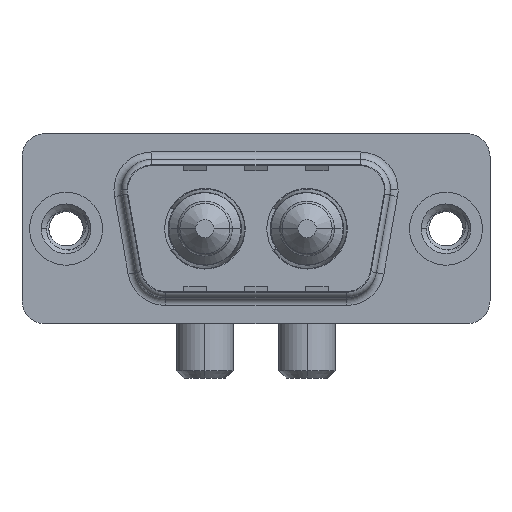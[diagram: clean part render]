
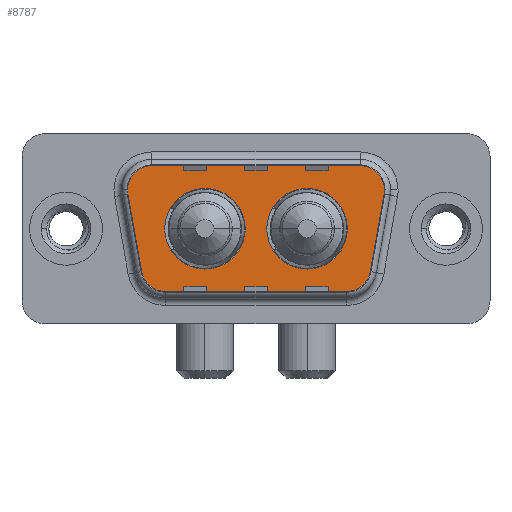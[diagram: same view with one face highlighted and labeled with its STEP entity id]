
A CAD part, top view. The second image highlights one B-rep face of the part: STEP entity #8787.
In plain terms, the highlighted planar face has unit normal (0, 0, 1).
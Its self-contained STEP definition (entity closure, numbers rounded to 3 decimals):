
#84 = CARTESIAN_POINT ( 'NONE',  ( 9.14, 0., 0. ) ) ;
#316 = LINE ( 'NONE', #6560, #7361 ) ;
#376 = CIRCLE ( 'NONE', #4851, 2.65 ) ;
#379 = DIRECTION ( 'NONE',  ( 0., 0., 1. ) ) ;
#532 = VERTEX_POINT ( 'NONE', #5671 ) ;
#815 = VECTOR ( 'NONE', #4176, 1000. ) ;
#820 = EDGE_CURVE ( 'NONE', #9684, #3343, #3651, .T. ) ;
#829 = EDGE_LOOP ( 'NONE', ( #10375, #3904, #11262, #5884, #11087, #3032, #9886, #11338, #3452 ) ) ;
#859 = DIRECTION ( 'NONE',  ( -1., 0., 0. ) ) ;
#915 = DIRECTION ( 'NONE',  ( 0., 0., 1. ) ) ;
#1034 = DIRECTION ( 'NONE',  ( 1., 0., 0. ) ) ;
#1186 = CARTESIAN_POINT ( 'NONE',  ( 5.436, 4.9, 0. ) ) ;
#1295 = EDGE_CURVE ( 'NONE', #2386, #5012, #4028, .T. ) ;
#1323 = CIRCLE ( 'NONE', #1509, 2.65 ) ;
#1374 = CARTESIAN_POINT ( 'NONE',  ( 3.466, 2.553, 0. ) ) ;
#1493 = ORIENTED_EDGE ( 'NONE', *, *, #3685, .F. ) ;
#1509 = AXIS2_PLACEMENT_3D ( 'NONE', #84, #6387, #7388 ) ;
#1539 = AXIS2_PLACEMENT_3D ( 'NONE', #5334, #1946, #9095 ) ;
#1560 = VECTOR ( 'NONE', #4746, 1000. ) ;
#1610 = DIRECTION ( 'NONE',  ( 0., 0., 1. ) ) ;
#1742 = CARTESIAN_POINT ( 'NONE',  ( 18.541, -2.9, 0. ) ) ;
#1842 = ORIENTED_EDGE ( 'NONE', *, *, #2055, .F. ) ;
#1946 = DIRECTION ( 'NONE',  ( 0., 0., 1. ) ) ;
#2055 = EDGE_CURVE ( 'NONE', #5024, #3481, #6381, .T. ) ;
#2069 = CARTESIAN_POINT ( 'NONE',  ( 19.564, 4.9, 0. ) ) ;
#2107 = AXIS2_PLACEMENT_3D ( 'NONE', #9787, #4604, #9852 ) ;
#2122 = EDGE_CURVE ( 'NONE', #532, #2526, #6026, .T. ) ;
#2143 = CARTESIAN_POINT ( 'NONE',  ( 9.14, 0., 0. ) ) ;
#2169 = AXIS2_PLACEMENT_3D ( 'NONE', #5074, #11203, #11319 ) ;
#2353 = CARTESIAN_POINT ( 'NONE',  ( 13.21, 0., 0. ) ) ;
#2386 = VERTEX_POINT ( 'NONE', #3941 ) ;
#2468 = AXIS2_PLACEMENT_3D ( 'NONE', #6372, #5561, #8194 ) ;
#2526 = VERTEX_POINT ( 'NONE', #11524 ) ;
#2695 = EDGE_CURVE ( 'NONE', #7485, #532, #4625, .T. ) ;
#3032 = ORIENTED_EDGE ( 'NONE', *, *, #2122, .T. ) ;
#3070 = LINE ( 'NONE', #1374, #7438 ) ;
#3191 = CARTESIAN_POINT ( 'NONE',  ( 21.534, 2.553, 0. ) ) ;
#3250 = ORIENTED_EDGE ( 'NONE', *, *, #7340, .F. ) ;
#3343 = VERTEX_POINT ( 'NONE', #10043 ) ;
#3402 = EDGE_LOOP ( 'NONE', ( #8997, #3250 ) ) ;
#3452 = ORIENTED_EDGE ( 'NONE', *, *, #10822, .T. ) ;
#3481 = VERTEX_POINT ( 'NONE', #2353 ) ;
#3567 = CIRCLE ( 'NONE', #8812, 2. ) ;
#3623 = CIRCLE ( 'NONE', #6228, 2. ) ;
#3651 = CIRCLE ( 'NONE', #2169, 2. ) ;
#3685 = EDGE_CURVE ( 'NONE', #3481, #5024, #9790, .T. ) ;
#3867 = VERTEX_POINT ( 'NONE', #7362 ) ;
#3904 = ORIENTED_EDGE ( 'NONE', *, *, #10394, .T. ) ;
#3907 = CARTESIAN_POINT ( 'NONE',  ( 6.49, 0., 0. ) ) ;
#3934 = CARTESIAN_POINT ( 'NONE',  ( 18.51, 0., 0. ) ) ;
#3941 = CARTESIAN_POINT ( 'NONE',  ( 21.534, 2.553, 0. ) ) ;
#4028 = CIRCLE ( 'NONE', #11345, 2. ) ;
#4176 = DIRECTION ( 'NONE',  ( 0.174, 0.985, 0. ) ) ;
#4476 = DIRECTION ( 'NONE',  ( -1., 0., 0. ) ) ;
#4604 = DIRECTION ( 'NONE',  ( 0., 0., 1. ) ) ;
#4625 = LINE ( 'NONE', #1186, #1560 ) ;
#4746 = DIRECTION ( 'NONE',  ( -1., 0., 0. ) ) ;
#4851 = AXIS2_PLACEMENT_3D ( 'NONE', #2143, #379, #5706 ) ;
#5012 = VERTEX_POINT ( 'NONE', #7679 ) ;
#5024 = VERTEX_POINT ( 'NONE', #3934 ) ;
#5029 = EDGE_CURVE ( 'NONE', #2526, #3867, #3070, .T. ) ;
#5074 = CARTESIAN_POINT ( 'NONE',  ( 18.541, -2.9, 0. ) ) ;
#5130 = VERTEX_POINT ( 'NONE', #5503 ) ;
#5227 = DIRECTION ( 'NONE',  ( -1., 0., 0. ) ) ;
#5334 = CARTESIAN_POINT ( 'NONE',  ( 15.86, 0., 0. ) ) ;
#5364 = CARTESIAN_POINT ( 'NONE',  ( 19.564, 2.9, 0. ) ) ;
#5503 = CARTESIAN_POINT ( 'NONE',  ( 11.79, 0., 0. ) ) ;
#5561 = DIRECTION ( 'NONE',  ( 0., 0., 1. ) ) ;
#5671 = CARTESIAN_POINT ( 'NONE',  ( 5.436, 4.9, 0. ) ) ;
#5688 = EDGE_LOOP ( 'NONE', ( #1842, #1493 ) ) ;
#5706 = DIRECTION ( 'NONE',  ( 1., 0., 0. ) ) ;
#5884 = ORIENTED_EDGE ( 'NONE', *, *, #10218, .T. ) ;
#6026 = CIRCLE ( 'NONE', #2468, 2. ) ;
#6163 = CARTESIAN_POINT ( 'NONE',  ( 19.564, 2.9, 0. ) ) ;
#6228 = AXIS2_PLACEMENT_3D ( 'NONE', #5364, #915, #4476 ) ;
#6372 = CARTESIAN_POINT ( 'NONE',  ( 5.436, 2.9, 0. ) ) ;
#6381 = CIRCLE ( 'NONE', #1539, 2.65 ) ;
#6387 = DIRECTION ( 'NONE',  ( 0., 0., 1. ) ) ;
#6560 = CARTESIAN_POINT ( 'NONE',  ( 6.459, -4.9, 0. ) ) ;
#7049 = FACE_BOUND ( 'NONE', #5688, .T. ) ;
#7107 = EDGE_CURVE ( 'NONE', #5130, #7790, #376, .T. ) ;
#7249 = CARTESIAN_POINT ( 'NONE',  ( 18.541, -4.9, 0. ) ) ;
#7340 = EDGE_CURVE ( 'NONE', #7790, #5130, #1323, .T. ) ;
#7361 = VECTOR ( 'NONE', #10169, 1000. ) ;
#7362 = CARTESIAN_POINT ( 'NONE',  ( 4.489, -3.247, 0. ) ) ;
#7388 = DIRECTION ( 'NONE',  ( 1., 0., 0. ) ) ;
#7438 = VECTOR ( 'NONE', #11282, 1000. ) ;
#7485 = VERTEX_POINT ( 'NONE', #2069 ) ;
#7679 = CARTESIAN_POINT ( 'NONE',  ( 21.564, 2.9, 0. ) ) ;
#7693 = LINE ( 'NONE', #3191, #815 ) ;
#7790 = VERTEX_POINT ( 'NONE', #3907 ) ;
#7879 = DIRECTION ( 'NONE',  ( 0., 0., 1. ) ) ;
#8176 = EDGE_CURVE ( 'NONE', #3867, #9961, #3567, .T. ) ;
#8194 = DIRECTION ( 'NONE',  ( 1., 0., 0. ) ) ;
#8768 = CARTESIAN_POINT ( 'NONE',  ( 6.459, -2.9, 0. ) ) ;
#8787 = ADVANCED_FACE ( 'NONE', ( #7049, #10780, #10657 ), #9892, .T. ) ;
#8812 = AXIS2_PLACEMENT_3D ( 'NONE', #8768, #7879, #859 ) ;
#8997 = ORIENTED_EDGE ( 'NONE', *, *, #7107, .F. ) ;
#9095 = DIRECTION ( 'NONE',  ( 1., 0., 0. ) ) ;
#9684 = VERTEX_POINT ( 'NONE', #7249 ) ;
#9787 = CARTESIAN_POINT ( 'NONE',  ( 15.86, 0., 0. ) ) ;
#9790 = CIRCLE ( 'NONE', #2107, 2.65 ) ;
#9852 = DIRECTION ( 'NONE',  ( 1., 0., 0. ) ) ;
#9886 = ORIENTED_EDGE ( 'NONE', *, *, #5029, .T. ) ;
#9892 = PLANE ( 'NONE',  #11090 ) ;
#9961 = VERTEX_POINT ( 'NONE', #11369 ) ;
#10043 = CARTESIAN_POINT ( 'NONE',  ( 20.511, -3.247, 0. ) ) ;
#10169 = DIRECTION ( 'NONE',  ( 1., 0., 0. ) ) ;
#10218 = EDGE_CURVE ( 'NONE', #5012, #7485, #3623, .T. ) ;
#10375 = ORIENTED_EDGE ( 'NONE', *, *, #820, .T. ) ;
#10394 = EDGE_CURVE ( 'NONE', #3343, #2386, #7693, .T. ) ;
#10605 = DIRECTION ( 'NONE',  ( 0., 0., 1. ) ) ;
#10657 = FACE_OUTER_BOUND ( 'NONE', #829, .T. ) ;
#10780 = FACE_BOUND ( 'NONE', #3402, .T. ) ;
#10822 = EDGE_CURVE ( 'NONE', #9961, #9684, #316, .T. ) ;
#11087 = ORIENTED_EDGE ( 'NONE', *, *, #2695, .T. ) ;
#11090 = AXIS2_PLACEMENT_3D ( 'NONE', #1742, #10605, #1034 ) ;
#11203 = DIRECTION ( 'NONE',  ( 0., 0., 1. ) ) ;
#11262 = ORIENTED_EDGE ( 'NONE', *, *, #1295, .T. ) ;
#11282 = DIRECTION ( 'NONE',  ( 0.174, -0.985, 0. ) ) ;
#11319 = DIRECTION ( 'NONE',  ( 1., 0., 0. ) ) ;
#11338 = ORIENTED_EDGE ( 'NONE', *, *, #8176, .T. ) ;
#11345 = AXIS2_PLACEMENT_3D ( 'NONE', #6163, #1610, #5227 ) ;
#11369 = CARTESIAN_POINT ( 'NONE',  ( 6.459, -4.9, 0. ) ) ;
#11524 = CARTESIAN_POINT ( 'NONE',  ( 3.466, 2.553, 0. ) ) ;
